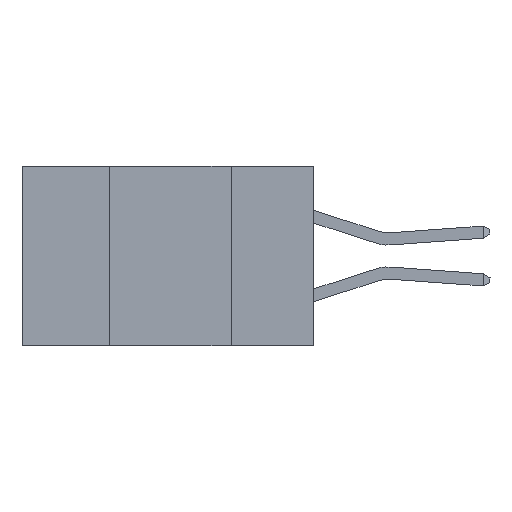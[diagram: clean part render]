
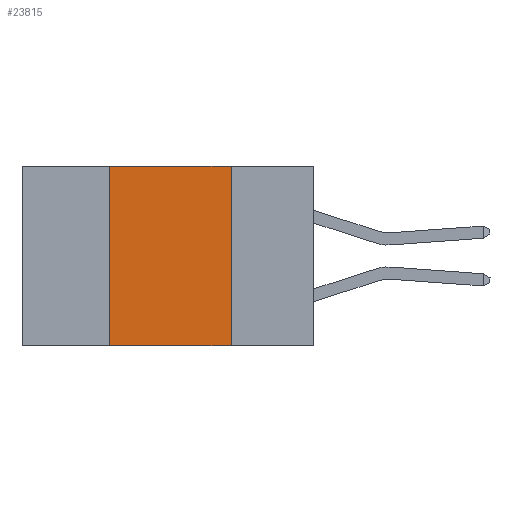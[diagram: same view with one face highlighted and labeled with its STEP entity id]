
A CAD part, left-side view. The second image highlights one B-rep face of the part: STEP entity #23815.
In plain terms, the highlighted planar face has unit normal (-1, 0, 0).
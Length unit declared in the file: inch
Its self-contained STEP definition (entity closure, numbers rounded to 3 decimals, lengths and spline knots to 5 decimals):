
#243 = VERTEX_POINT ( 'NONE', #23788 ) ;
#523 = EDGE_CURVE ( 'NONE', #15366, #18044, #26483, .T. ) ;
#717 = EDGE_CURVE ( 'NONE', #243, #18044, #10520, .T. ) ;
#1017 = CARTESIAN_POINT ( 'NONE',  ( 0., 0.6, 0. ) ) ;
#4622 = EDGE_LOOP ( 'NONE', ( #21739, #31679, #25578, #15271 ) ) ;
#7914 = AXIS2_PLACEMENT_3D ( 'NONE', #20667, #23079, #33533 ) ;
#8105 = LINE ( 'NONE', #1017, #30994 ) ;
#9317 = CARTESIAN_POINT ( 'NONE',  ( 0., 0.6, -0.37 ) ) ;
#10520 = LINE ( 'NONE', #9317, #21567 ) ;
#11515 = DIRECTION ( 'NONE',  ( 0., 0., -1. ) ) ;
#13988 = DIRECTION ( 'NONE',  ( 0., -1., 0. ) ) ;
#13991 = LINE ( 'NONE', #27715, #20930 ) ;
#15271 = ORIENTED_EDGE ( 'NONE', *, *, #717, .T. ) ;
#15366 = VERTEX_POINT ( 'NONE', #24510 ) ;
#17558 = EDGE_CURVE ( 'NONE', #243, #26477, #13991, .T. ) ;
#18044 = VERTEX_POINT ( 'NONE', #30226 ) ;
#20667 = CARTESIAN_POINT ( 'NONE',  ( 0., 0.6, 0. ) ) ;
#20930 = VECTOR ( 'NONE', #22489, 39.37008 ) ;
#21567 = VECTOR ( 'NONE', #22726, 39.37008 ) ;
#21739 = ORIENTED_EDGE ( 'NONE', *, *, #523, .F. ) ;
#22489 = DIRECTION ( 'NONE',  ( 0., 0., 1. ) ) ;
#22726 = DIRECTION ( 'NONE',  ( 0., -1., 0. ) ) ;
#23079 = DIRECTION ( 'NONE',  ( 1., 0., 0. ) ) ;
#23788 = CARTESIAN_POINT ( 'NONE',  ( 0., 0.42, -0.37 ) ) ;
#23815 = ADVANCED_FACE ( 'NONE', ( #29293 ), #25576, .F. ) ;
#24510 = CARTESIAN_POINT ( 'NONE',  ( 0., 0.17, 0. ) ) ;
#25576 = PLANE ( 'NONE',  #7914 ) ;
#25578 = ORIENTED_EDGE ( 'NONE', *, *, #17558, .F. ) ;
#26105 = VECTOR ( 'NONE', #11515, 39.37008 ) ;
#26477 = VERTEX_POINT ( 'NONE', #27471 ) ;
#26483 = LINE ( 'NONE', #29689, #26105 ) ;
#27471 = CARTESIAN_POINT ( 'NONE',  ( 0., 0.42, 0. ) ) ;
#27506 = EDGE_CURVE ( 'NONE', #26477, #15366, #8105, .T. ) ;
#27715 = CARTESIAN_POINT ( 'NONE',  ( 0., 0.42, 0. ) ) ;
#29293 = FACE_OUTER_BOUND ( 'NONE', #4622, .T. ) ;
#29689 = CARTESIAN_POINT ( 'NONE',  ( 0., 0.17, 0. ) ) ;
#30226 = CARTESIAN_POINT ( 'NONE',  ( 0., 0.17, -0.37 ) ) ;
#30994 = VECTOR ( 'NONE', #13988, 39.37008 ) ;
#31679 = ORIENTED_EDGE ( 'NONE', *, *, #27506, .F. ) ;
#33533 = DIRECTION ( 'NONE',  ( 0., 0., -1. ) ) ;
